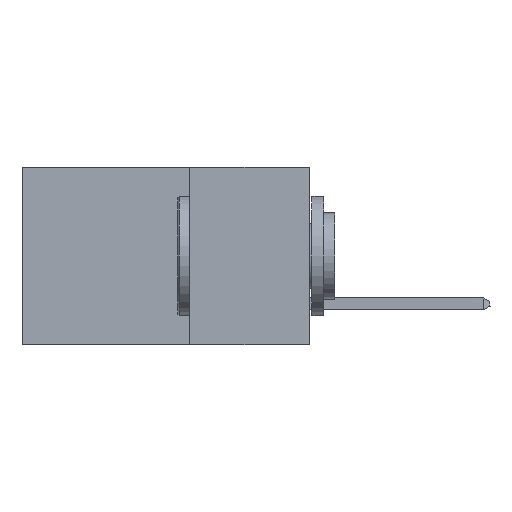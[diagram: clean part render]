
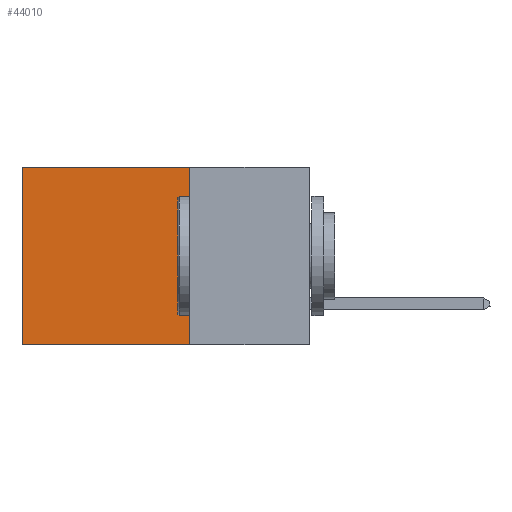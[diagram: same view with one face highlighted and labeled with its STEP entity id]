
A CAD part, left-side view. The second image highlights one B-rep face of the part: STEP entity #44010.
In plain terms, the highlighted planar face has unit normal (-1, 0, 0).
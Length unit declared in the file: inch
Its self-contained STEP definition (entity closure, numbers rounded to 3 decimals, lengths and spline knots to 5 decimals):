
#880 = ORIENTED_EDGE ( 'NONE', *, *, #36162, .T. ) ;
#2399 = ORIENTED_EDGE ( 'NONE', *, *, #13420, .T. ) ;
#3114 = DIRECTION ( 'NONE',  ( 1., 0., 0. ) ) ;
#3158 = FACE_OUTER_BOUND ( 'NONE', #9043, .T. ) ;
#3410 = DIRECTION ( 'NONE',  ( 0., 0., -1. ) ) ;
#3930 = VECTOR ( 'NONE', #20591, 39.37008 ) ;
#4267 = DIRECTION ( 'NONE',  ( 0., 0., -1. ) ) ;
#4502 = VERTEX_POINT ( 'NONE', #27077 ) ;
#5025 = EDGE_CURVE ( 'NONE', #22356, #4502, #29450, .T. ) ;
#9043 = EDGE_LOOP ( 'NONE', ( #880, #31357, #38250, #2399 ) ) ;
#9311 = VERTEX_POINT ( 'NONE', #43898 ) ;
#9705 = CARTESIAN_POINT ( 'NONE',  ( 0.2875, 0.6, 0. ) ) ;
#9713 = LINE ( 'NONE', #32089, #25324 ) ;
#9868 = DIRECTION ( 'NONE',  ( 0., 1., 0. ) ) ;
#10463 = LINE ( 'NONE', #30894, #19148 ) ;
#13420 = EDGE_CURVE ( 'NONE', #9311, #32551, #10463, .T. ) ;
#13957 = PLANE ( 'NONE',  #43692 ) ;
#14308 = CARTESIAN_POINT ( 'NONE',  ( 0.2875, 0.25, -0.37 ) ) ;
#19148 = VECTOR ( 'NONE', #30607, 39.37008 ) ;
#20591 = DIRECTION ( 'NONE',  ( 0., 0., -1. ) ) ;
#22356 = VERTEX_POINT ( 'NONE', #14308 ) ;
#25324 = VECTOR ( 'NONE', #4267, 39.37008 ) ;
#27077 = CARTESIAN_POINT ( 'NONE',  ( 0.2875, 0.6, -0.37 ) ) ;
#28232 = LINE ( 'NONE', #28688, #3930 ) ;
#28688 = CARTESIAN_POINT ( 'NONE',  ( 0.2875, 0.25, 0. ) ) ;
#29450 = LINE ( 'NONE', #30559, #40222 ) ;
#30559 = CARTESIAN_POINT ( 'NONE',  ( 0.2875, 0.25, -0.37 ) ) ;
#30607 = DIRECTION ( 'NONE',  ( 0., 1., 0. ) ) ;
#30894 = CARTESIAN_POINT ( 'NONE',  ( 0.2875, 0.25, 0. ) ) ;
#31357 = ORIENTED_EDGE ( 'NONE', *, *, #5025, .F. ) ;
#31729 = EDGE_CURVE ( 'NONE', #9311, #22356, #28232, .T. ) ;
#32089 = CARTESIAN_POINT ( 'NONE',  ( 0.2875, 0.6, 0. ) ) ;
#32551 = VERTEX_POINT ( 'NONE', #9705 ) ;
#36162 = EDGE_CURVE ( 'NONE', #32551, #4502, #9713, .T. ) ;
#38250 = ORIENTED_EDGE ( 'NONE', *, *, #31729, .F. ) ;
#40222 = VECTOR ( 'NONE', #9868, 39.37008 ) ;
#41124 = CARTESIAN_POINT ( 'NONE',  ( 0.2875, 0.25, 0. ) ) ;
#43692 = AXIS2_PLACEMENT_3D ( 'NONE', #41124, #3114, #3410 ) ;
#43898 = CARTESIAN_POINT ( 'NONE',  ( 0.2875, 0.25, 0. ) ) ;
#44010 = ADVANCED_FACE ( 'NONE', ( #3158 ), #13957, .F. ) ;
